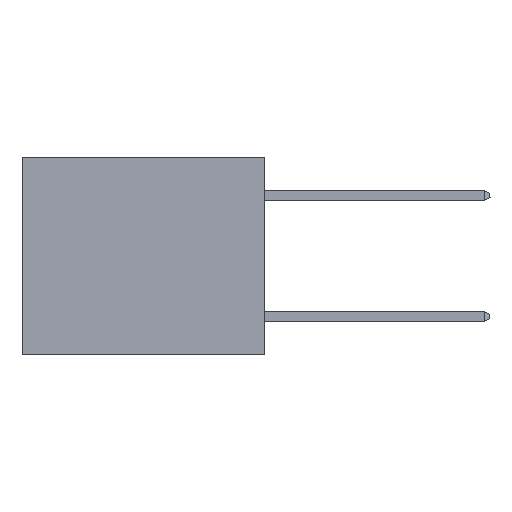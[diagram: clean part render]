
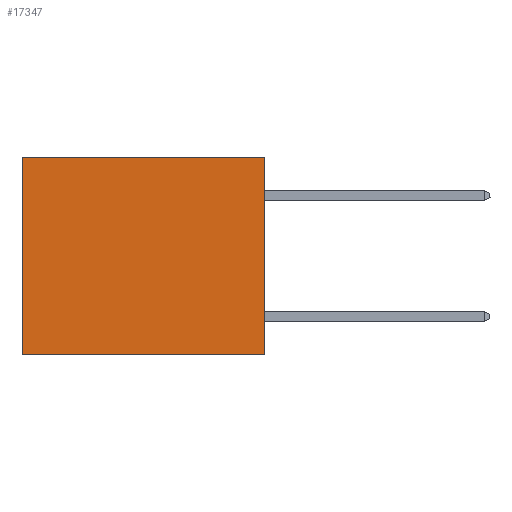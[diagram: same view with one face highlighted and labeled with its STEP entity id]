
A CAD part, left-side view. The second image highlights one B-rep face of the part: STEP entity #17347.
In plain terms, the highlighted planar face has unit normal (-1, 0, 0).
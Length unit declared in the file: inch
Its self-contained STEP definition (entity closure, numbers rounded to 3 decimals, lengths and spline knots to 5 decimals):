
#529 = VECTOR ( 'NONE', #17730, 39.37008 ) ;
#1030 = LINE ( 'NONE', #15714, #1749 ) ;
#1749 = VECTOR ( 'NONE', #13468, 39.37008 ) ;
#2124 = EDGE_CURVE ( 'NONE', #9059, #22809, #6931, .T. ) ;
#2177 = DIRECTION ( 'NONE',  ( 0., 1., 0. ) ) ;
#2591 = EDGE_CURVE ( 'NONE', #8774, #9059, #1030, .T. ) ;
#2679 = VECTOR ( 'NONE', #11985, 39.37008 ) ;
#3282 = ORIENTED_EDGE ( 'NONE', *, *, #17634, .T. ) ;
#3961 = CARTESIAN_POINT ( 'NONE',  ( 0.3165, 0.6, -0.49 ) ) ;
#3974 = CARTESIAN_POINT ( 'NONE',  ( 0.3165, 0., -0.49 ) ) ;
#4017 = DIRECTION ( 'NONE',  ( 1., 0., 0. ) ) ;
#4224 = ORIENTED_EDGE ( 'NONE', *, *, #2124, .F. ) ;
#6695 = VERTEX_POINT ( 'NONE', #26479 ) ;
#6931 = LINE ( 'NONE', #18987, #19025 ) ;
#7716 = CARTESIAN_POINT ( 'NONE',  ( 0.3165, 0.6, -0.49 ) ) ;
#8774 = VERTEX_POINT ( 'NONE', #30167 ) ;
#8937 = FACE_OUTER_BOUND ( 'NONE', #25890, .T. ) ;
#9059 = VERTEX_POINT ( 'NONE', #3974 ) ;
#11985 = DIRECTION ( 'NONE',  ( 0., 1., 0. ) ) ;
#13468 = DIRECTION ( 'NONE',  ( 0., 0., -1. ) ) ;
#13778 = ORIENTED_EDGE ( 'NONE', *, *, #16920, .T. ) ;
#15115 = LINE ( 'NONE', #25921, #2679 ) ;
#15711 = AXIS2_PLACEMENT_3D ( 'NONE', #20724, #4017, #25546 ) ;
#15714 = CARTESIAN_POINT ( 'NONE',  ( 0.3165, 0., -0.49 ) ) ;
#16920 = EDGE_CURVE ( 'NONE', #6695, #22809, #19575, .T. ) ;
#17347 = ADVANCED_FACE ( 'NONE', ( #8937 ), #27700, .F. ) ;
#17634 = EDGE_CURVE ( 'NONE', #8774, #6695, #15115, .T. ) ;
#17730 = DIRECTION ( 'NONE',  ( 0., 0., -1. ) ) ;
#18987 = CARTESIAN_POINT ( 'NONE',  ( 0.3165, 0., -0.49 ) ) ;
#19025 = VECTOR ( 'NONE', #2177, 39.37008 ) ;
#19575 = LINE ( 'NONE', #3961, #529 ) ;
#20724 = CARTESIAN_POINT ( 'NONE',  ( 0.3165, 0., -0.49 ) ) ;
#22809 = VERTEX_POINT ( 'NONE', #7716 ) ;
#25546 = DIRECTION ( 'NONE',  ( 0., 0., -1. ) ) ;
#25890 = EDGE_LOOP ( 'NONE', ( #13778, #4224, #26666, #3282 ) ) ;
#25921 = CARTESIAN_POINT ( 'NONE',  ( 0.3165, 0., 0. ) ) ;
#26479 = CARTESIAN_POINT ( 'NONE',  ( 0.3165, 0.6, 0. ) ) ;
#26666 = ORIENTED_EDGE ( 'NONE', *, *, #2591, .F. ) ;
#27700 = PLANE ( 'NONE',  #15711 ) ;
#30167 = CARTESIAN_POINT ( 'NONE',  ( 0.3165, 0., 0. ) ) ;
